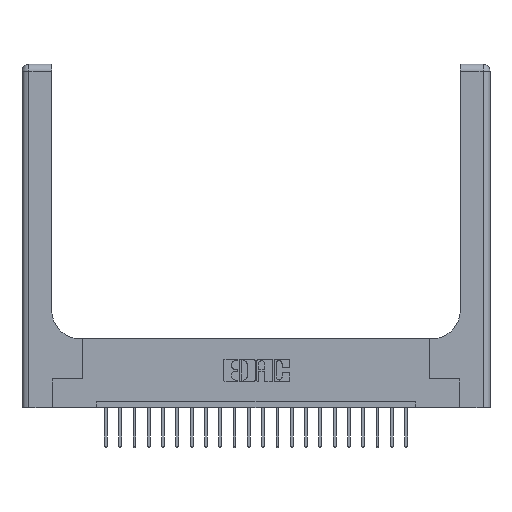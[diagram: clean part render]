
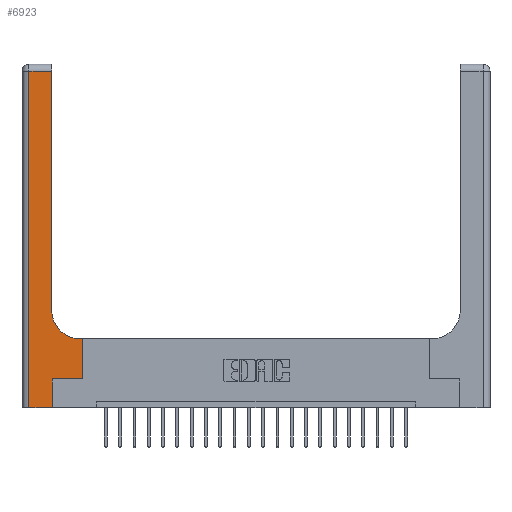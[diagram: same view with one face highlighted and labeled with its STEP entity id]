
A CAD part, top view. The second image highlights one B-rep face of the part: STEP entity #6923.
In plain terms, the highlighted planar face has unit normal (0, 0, 1).
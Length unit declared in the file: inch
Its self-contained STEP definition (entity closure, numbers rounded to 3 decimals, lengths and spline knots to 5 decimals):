
#12 = FACE_OUTER_BOUND ( 'NONE', #12748, .T. ) ;
#138 = AXIS2_PLACEMENT_3D ( 'NONE', #16907, #8700, #20245 ) ;
#576 = EDGE_CURVE ( 'NONE', #8541, #12684, #19369, .T. ) ;
#686 = LINE ( 'NONE', #7471, #12603 ) ;
#798 = EDGE_CURVE ( 'NONE', #6515, #14077, #686, .T. ) ;
#1115 = VERTEX_POINT ( 'NONE', #2096 ) ;
#1461 = LINE ( 'NONE', #16462, #18348 ) ;
#2012 = CARTESIAN_POINT ( 'NONE',  ( 0.26, 2.94, 0.37 ) ) ;
#2096 = CARTESIAN_POINT ( 'NONE',  ( 0.265, 0.25, 0.37 ) ) ;
#2371 = DIRECTION ( 'NONE',  ( -1., 0., 0. ) ) ;
#2573 = ORIENTED_EDGE ( 'NONE', *, *, #19930, .T. ) ;
#3026 = CARTESIAN_POINT ( 'NONE',  ( 0.265, 0.25, 0.37 ) ) ;
#3070 = VECTOR ( 'NONE', #14484, 39.37008 ) ;
#3159 = EDGE_CURVE ( 'NONE', #1115, #6294, #11452, .T. ) ;
#3623 = LINE ( 'NONE', #20736, #4136 ) ;
#4136 = VECTOR ( 'NONE', #8520, 39.37008 ) ;
#4227 = CARTESIAN_POINT ( 'NONE',  ( 0.528, 0.25, 0.37 ) ) ;
#4500 = ORIENTED_EDGE ( 'NONE', *, *, #11406, .T. ) ;
#4589 = DIRECTION ( 'NONE',  ( 0., 1., 0. ) ) ;
#5115 = VECTOR ( 'NONE', #17313, 39.37008 ) ;
#5353 = ORIENTED_EDGE ( 'NONE', *, *, #576, .T. ) ;
#5749 = CARTESIAN_POINT ( 'NONE',  ( 0.26, 0.85, 0.37 ) ) ;
#6072 = CARTESIAN_POINT ( 'NONE',  ( 0.06, 3., 0.37 ) ) ;
#6184 = EDGE_CURVE ( 'NONE', #14077, #17579, #14654, .T. ) ;
#6294 = VERTEX_POINT ( 'NONE', #4227 ) ;
#6515 = VERTEX_POINT ( 'NONE', #12060 ) ;
#6923 = ADVANCED_FACE ( 'NONE', ( #12 ), #16793, .F. ) ;
#7008 = CARTESIAN_POINT ( 'NONE',  ( 0.265, 0., 0.37 ) ) ;
#7378 = EDGE_CURVE ( 'NONE', #16436, #1115, #20779, .T. ) ;
#7471 = CARTESIAN_POINT ( 'NONE',  ( 0.26, 0.6, 0.37 ) ) ;
#7957 = DIRECTION ( 'NONE',  ( 0., -1., 0. ) ) ;
#8131 = DIRECTION ( 'NONE',  ( 1., 0., 0. ) ) ;
#8520 = DIRECTION ( 'NONE',  ( 0., 1., 0. ) ) ;
#8541 = VERTEX_POINT ( 'NONE', #2012 ) ;
#8700 = DIRECTION ( 'NONE',  ( 0., 0., -1. ) ) ;
#8941 = CARTESIAN_POINT ( 'NONE',  ( 0., 2.94, 0.37 ) ) ;
#8945 = ORIENTED_EDGE ( 'NONE', *, *, #11887, .T. ) ;
#10137 = CARTESIAN_POINT ( 'NONE',  ( 0.06, 2.94, 0.37 ) ) ;
#11406 = EDGE_CURVE ( 'NONE', #6294, #6515, #1461, .T. ) ;
#11452 = LINE ( 'NONE', #3026, #20656 ) ;
#11670 = DIRECTION ( 'NONE',  ( 1., 0., 0. ) ) ;
#11887 = EDGE_CURVE ( 'NONE', #17579, #8541, #3623, .T. ) ;
#12060 = CARTESIAN_POINT ( 'NONE',  ( 0.528, 0.6, 0.37 ) ) ;
#12603 = VECTOR ( 'NONE', #2371, 39.37008 ) ;
#12684 = VERTEX_POINT ( 'NONE', #10137 ) ;
#12748 = EDGE_LOOP ( 'NONE', ( #8945, #5353, #20000, #2573, #16999, #12956, #4500, #16101, #20351 ) ) ;
#12956 = ORIENTED_EDGE ( 'NONE', *, *, #3159, .T. ) ;
#14045 = CARTESIAN_POINT ( 'NONE',  ( 0., 0., 0.37 ) ) ;
#14077 = VERTEX_POINT ( 'NONE', #14561 ) ;
#14276 = VECTOR ( 'NONE', #20835, 39.37008 ) ;
#14484 = DIRECTION ( 'NONE',  ( -1., 0., 0. ) ) ;
#14561 = CARTESIAN_POINT ( 'NONE',  ( 0.51, 0.6, 0.37 ) ) ;
#14654 = CIRCLE ( 'NONE', #20336, 0.25 ) ;
#14806 = EDGE_CURVE ( 'NONE', #12684, #14920, #21299, .T. ) ;
#14920 = VERTEX_POINT ( 'NONE', #21948 ) ;
#15546 = VECTOR ( 'NONE', #7957, 39.37008 ) ;
#15698 = LINE ( 'NONE', #14045, #14276 ) ;
#16101 = ORIENTED_EDGE ( 'NONE', *, *, #798, .T. ) ;
#16436 = VERTEX_POINT ( 'NONE', #21526 ) ;
#16462 = CARTESIAN_POINT ( 'NONE',  ( 0.528, 0.25, 0.37 ) ) ;
#16793 = PLANE ( 'NONE',  #138 ) ;
#16907 = CARTESIAN_POINT ( 'NONE',  ( 0., 3., 0.37 ) ) ;
#16999 = ORIENTED_EDGE ( 'NONE', *, *, #7378, .T. ) ;
#17313 = DIRECTION ( 'NONE',  ( 0., 1., 0. ) ) ;
#17579 = VERTEX_POINT ( 'NONE', #5749 ) ;
#18348 = VECTOR ( 'NONE', #4589, 39.37008 ) ;
#19369 = LINE ( 'NONE', #8941, #3070 ) ;
#19930 = EDGE_CURVE ( 'NONE', #14920, #16436, #15698, .T. ) ;
#20000 = ORIENTED_EDGE ( 'NONE', *, *, #14806, .T. ) ;
#20124 = CARTESIAN_POINT ( 'NONE',  ( 0.51, 0.85, 0.37 ) ) ;
#20237 = DIRECTION ( 'NONE',  ( 0., 0., -1. ) ) ;
#20245 = DIRECTION ( 'NONE',  ( -1., 0., 0. ) ) ;
#20336 = AXIS2_PLACEMENT_3D ( 'NONE', #20124, #20237, #11670 ) ;
#20351 = ORIENTED_EDGE ( 'NONE', *, *, #6184, .T. ) ;
#20656 = VECTOR ( 'NONE', #8131, 39.37008 ) ;
#20736 = CARTESIAN_POINT ( 'NONE',  ( 0.26, 3., 0.37 ) ) ;
#20779 = LINE ( 'NONE', #7008, #5115 ) ;
#20835 = DIRECTION ( 'NONE',  ( 1., 0., 0. ) ) ;
#21299 = LINE ( 'NONE', #6072, #15546 ) ;
#21526 = CARTESIAN_POINT ( 'NONE',  ( 0.265, 0., 0.37 ) ) ;
#21948 = CARTESIAN_POINT ( 'NONE',  ( 0.06, 0., 0.37 ) ) ;
